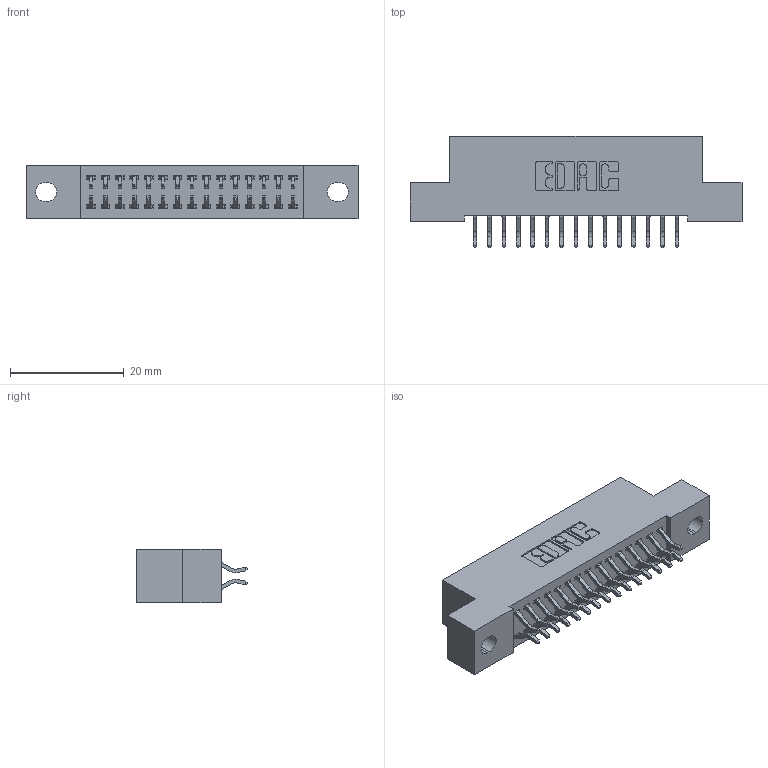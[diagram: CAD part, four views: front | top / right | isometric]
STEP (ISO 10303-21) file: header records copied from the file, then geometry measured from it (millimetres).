
FILE_DESCRIPTION (( 'STEP AP203' ), '1' );
FILE_NAME ('342-030-556-202.STEP', '2018-08-11T15:47:47', ( '' ), ( '' ), 'SwSTEP 2.0', 'SolidWorks 2016', '' );
FILE_SCHEMA (( 'CONFIG_CONTROL_DESIGN' ));
Length unit declared in the file: inch
Products named in the file (3): 342-030-556-202; 342 Part_.128 Slot; 345-292-001_556 Tail
Assembly tree (31 placements, depth 2):
  342-030-556-202
    342 Part_.128 Slot
    345-292-001_556 Tail  x30
Bounding box: 58.42 x 19.58 x 9.4 mm (x, y, z)
Volume: 5068.3 mm3; surface area: 7315 mm2
Topology: 31 solids, 31 shells, 1854 faces, 5501 edges, 3626 vertices
Faces by surface type: plane 1270, cylinder 584
Entity records: 13365 total; most frequent: CARTESIAN_POINT 2262, ORIENTED_EDGE 2186, DIRECTION 1969, EDGE_CURVE 1093, LINE 957, VECTOR 957, VERTEX_POINT 726, AXIS2_PLACEMENT_3D 506
